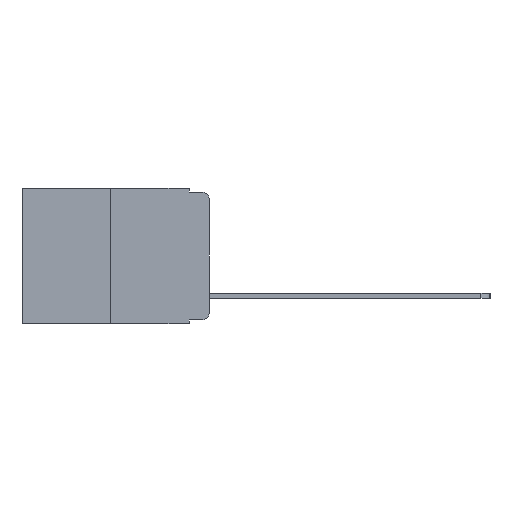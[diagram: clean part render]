
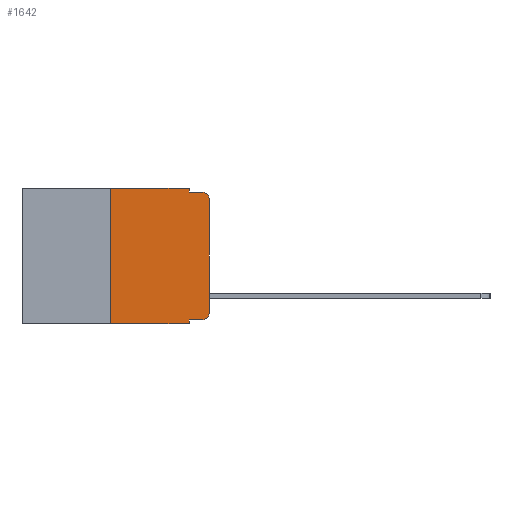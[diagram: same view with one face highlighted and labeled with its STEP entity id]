
A CAD part, left-side view. The second image highlights one B-rep face of the part: STEP entity #1642.
In plain terms, the highlighted planar face has unit normal (-1, 0, 0).
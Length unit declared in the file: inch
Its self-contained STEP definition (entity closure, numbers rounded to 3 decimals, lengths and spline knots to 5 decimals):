
#198 = DIRECTION ( 'NONE',  ( 0., 0., -1. ) ) ;
#395 = VERTEX_POINT ( 'NONE', #7830 ) ;
#402 = VERTEX_POINT ( 'NONE', #8906 ) ;
#483 = DIRECTION ( 'NONE',  ( 0., -1., 0. ) ) ;
#528 = VERTEX_POINT ( 'NONE', #6152 ) ;
#678 = VERTEX_POINT ( 'NONE', #5218 ) ;
#922 = CARTESIAN_POINT ( 'NONE',  ( 0., 0.051, 0. ) ) ;
#1320 = FACE_OUTER_BOUND ( 'NONE', #6845, .T. ) ;
#1335 = LINE ( 'NONE', #922, #14534 ) ;
#1355 = CARTESIAN_POINT ( 'NONE',  ( 0., 0.473, 0. ) ) ;
#1642 = ADVANCED_FACE ( 'NONE', ( #1320 ), #10017, .F. ) ;
#1952 = EDGE_CURVE ( 'NONE', #4983, #12308, #13268, .T. ) ;
#1988 = LINE ( 'NONE', #12639, #11645 ) ;
#2203 = DIRECTION ( 'NONE',  ( 0., 0., -1. ) ) ;
#2210 = DIRECTION ( 'NONE',  ( 1., 0., 0. ) ) ;
#2333 = CARTESIAN_POINT ( 'NONE',  ( 0., 0.473, -0.343 ) ) ;
#2533 = AXIS2_PLACEMENT_3D ( 'NONE', #7641, #8478, #8915 ) ;
#2892 = ORIENTED_EDGE ( 'NONE', *, *, #9573, .F. ) ;
#2943 = DIRECTION ( 'NONE',  ( 0., 0., 1. ) ) ;
#3277 = CARTESIAN_POINT ( 'NONE',  ( 0., 0.02, -0.333 ) ) ;
#3595 = VERTEX_POINT ( 'NONE', #14989 ) ;
#3808 = VERTEX_POINT ( 'NONE', #3277 ) ;
#3927 = VERTEX_POINT ( 'NONE', #14262 ) ;
#4212 = ORIENTED_EDGE ( 'NONE', *, *, #13527, .T. ) ;
#4983 = VERTEX_POINT ( 'NONE', #13053 ) ;
#5155 = ORIENTED_EDGE ( 'NONE', *, *, #12093, .T. ) ;
#5218 = CARTESIAN_POINT ( 'NONE',  ( 0., 0.051, -0.333 ) ) ;
#5361 = CIRCLE ( 'NONE', #13489, 0.02 ) ;
#5636 = VECTOR ( 'NONE', #15130, 39.37008 ) ;
#5823 = DIRECTION ( 'NONE',  ( 0., 0., -1. ) ) ;
#6152 = CARTESIAN_POINT ( 'NONE',  ( 0., 0.051, -0.01 ) ) ;
#6463 = ORIENTED_EDGE ( 'NONE', *, *, #13417, .T. ) ;
#6607 = ORIENTED_EDGE ( 'NONE', *, *, #9438, .T. ) ;
#6845 = EDGE_LOOP ( 'NONE', ( #4212, #6607, #9846, #10610, #12509, #2892, #15642, #15734, #5155, #6463 ) ) ;
#7641 = CARTESIAN_POINT ( 'NONE',  ( 0., 0.02, -0.03 ) ) ;
#7742 = CARTESIAN_POINT ( 'NONE',  ( 0., 0.051, 0. ) ) ;
#7746 = EDGE_CURVE ( 'NONE', #12308, #528, #14323, .T. ) ;
#7830 = CARTESIAN_POINT ( 'NONE',  ( 0., 0.02, -0.01 ) ) ;
#7841 = DIRECTION ( 'NONE',  ( -1., 0., 0. ) ) ;
#8024 = CIRCLE ( 'NONE', #2533, 0.02 ) ;
#8106 = CARTESIAN_POINT ( 'NONE',  ( 0., 0.051, -0.01 ) ) ;
#8156 = CARTESIAN_POINT ( 'NONE',  ( 0., 0.051, 0. ) ) ;
#8412 = VECTOR ( 'NONE', #8667, 39.37008 ) ;
#8478 = DIRECTION ( 'NONE',  ( -1., 0., 0. ) ) ;
#8602 = EDGE_CURVE ( 'NONE', #528, #395, #10594, .T. ) ;
#8667 = DIRECTION ( 'NONE',  ( 0., -1., 0. ) ) ;
#8749 = AXIS2_PLACEMENT_3D ( 'NONE', #1355, #2210, #5823 ) ;
#8755 = CARTESIAN_POINT ( 'NONE',  ( 0., 0.25, -0.343 ) ) ;
#8906 = CARTESIAN_POINT ( 'NONE',  ( 0., 0., -0.313 ) ) ;
#8915 = DIRECTION ( 'NONE',  ( 0., 0., -1. ) ) ;
#9362 = VERTEX_POINT ( 'NONE', #8755 ) ;
#9438 = EDGE_CURVE ( 'NONE', #3595, #395, #8024, .T. ) ;
#9460 = DIRECTION ( 'NONE',  ( 0., -1., 0. ) ) ;
#9573 = EDGE_CURVE ( 'NONE', #9362, #4983, #9799, .T. ) ;
#9799 = LINE ( 'NONE', #13997, #5636 ) ;
#9846 = ORIENTED_EDGE ( 'NONE', *, *, #8602, .F. ) ;
#10017 = PLANE ( 'NONE',  #8749 ) ;
#10032 = VECTOR ( 'NONE', #9460, 39.37008 ) ;
#10088 = VECTOR ( 'NONE', #2943, 39.37008 ) ;
#10418 = EDGE_CURVE ( 'NONE', #9362, #3927, #11705, .T. ) ;
#10594 = LINE ( 'NONE', #8106, #10962 ) ;
#10610 = ORIENTED_EDGE ( 'NONE', *, *, #7746, .F. ) ;
#10962 = VECTOR ( 'NONE', #483, 39.37008 ) ;
#11412 = DIRECTION ( 'NONE',  ( 0., -1., 0. ) ) ;
#11542 = VECTOR ( 'NONE', #14973, 39.37008 ) ;
#11645 = VECTOR ( 'NONE', #11412, 39.37008 ) ;
#11705 = LINE ( 'NONE', #2333, #8412 ) ;
#11738 = CARTESIAN_POINT ( 'NONE',  ( 0., 0., 0. ) ) ;
#12093 = EDGE_CURVE ( 'NONE', #678, #3808, #1988, .T. ) ;
#12308 = VERTEX_POINT ( 'NONE', #8156 ) ;
#12509 = ORIENTED_EDGE ( 'NONE', *, *, #1952, .F. ) ;
#12639 = CARTESIAN_POINT ( 'NONE',  ( 0., 0.051, -0.333 ) ) ;
#13053 = CARTESIAN_POINT ( 'NONE',  ( 0., 0.25, 0. ) ) ;
#13148 = CARTESIAN_POINT ( 'NONE',  ( 0., 0.473, 0. ) ) ;
#13268 = LINE ( 'NONE', #13148, #10032 ) ;
#13417 = EDGE_CURVE ( 'NONE', #3808, #402, #5361, .T. ) ;
#13489 = AXIS2_PLACEMENT_3D ( 'NONE', #15061, #7841, #198 ) ;
#13527 = EDGE_CURVE ( 'NONE', #402, #3595, #13690, .T. ) ;
#13690 = LINE ( 'NONE', #11738, #10088 ) ;
#13997 = CARTESIAN_POINT ( 'NONE',  ( 0., 0.25, 0. ) ) ;
#14262 = CARTESIAN_POINT ( 'NONE',  ( 0., 0.051, -0.343 ) ) ;
#14323 = LINE ( 'NONE', #7742, #11542 ) ;
#14493 = EDGE_CURVE ( 'NONE', #678, #3927, #1335, .T. ) ;
#14534 = VECTOR ( 'NONE', #2203, 39.37008 ) ;
#14973 = DIRECTION ( 'NONE',  ( 0., 0., -1. ) ) ;
#14989 = CARTESIAN_POINT ( 'NONE',  ( 0., 0., -0.03 ) ) ;
#15061 = CARTESIAN_POINT ( 'NONE',  ( 0., 0.02, -0.313 ) ) ;
#15130 = DIRECTION ( 'NONE',  ( 0., 0., 1. ) ) ;
#15642 = ORIENTED_EDGE ( 'NONE', *, *, #10418, .T. ) ;
#15734 = ORIENTED_EDGE ( 'NONE', *, *, #14493, .F. ) ;
